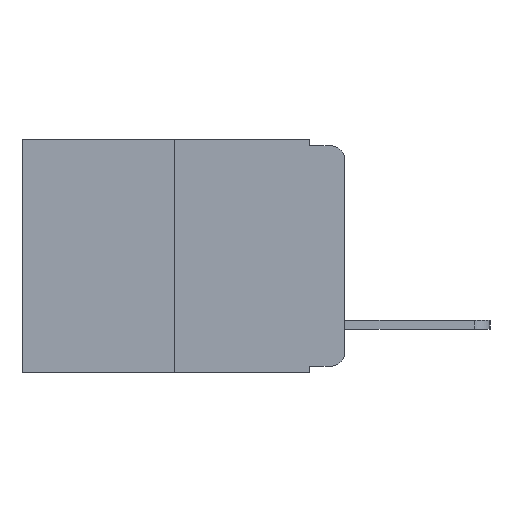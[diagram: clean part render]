
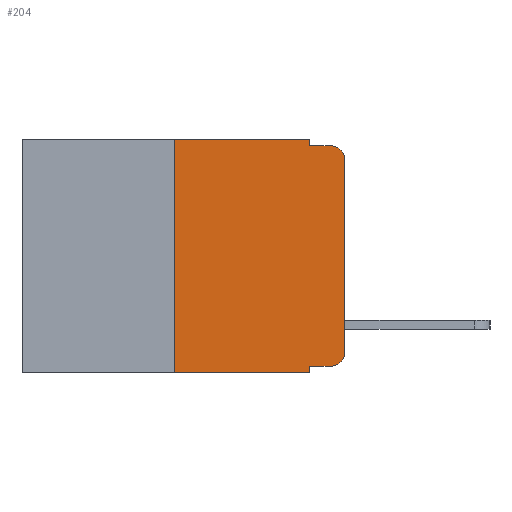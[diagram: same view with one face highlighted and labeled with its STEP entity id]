
A CAD part, left-side view. The second image highlights one B-rep face of the part: STEP entity #204.
In plain terms, the highlighted planar face has unit normal (-1, 0, 0).
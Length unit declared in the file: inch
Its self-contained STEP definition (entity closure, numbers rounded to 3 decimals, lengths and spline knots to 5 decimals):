
#204 = ADVANCED_FACE ( 'NONE', ( #9454 ), #4370, .F. ) ;
#456 = LINE ( 'NONE', #2460, #6495 ) ;
#551 = CARTESIAN_POINT ( 'NONE',  ( 0., 0.051, -0.333 ) ) ;
#660 = VERTEX_POINT ( 'NONE', #8153 ) ;
#873 = DIRECTION ( 'NONE',  ( 0., 0., -1. ) ) ;
#1065 = VERTEX_POINT ( 'NONE', #3341 ) ;
#1550 = VERTEX_POINT ( 'NONE', #4967 ) ;
#1679 = ORIENTED_EDGE ( 'NONE', *, *, #2929, .F. ) ;
#1696 = DIRECTION ( 'NONE',  ( -1., 0., 0. ) ) ;
#1979 = EDGE_CURVE ( 'NONE', #2777, #8733, #5225, .T. ) ;
#2117 = VECTOR ( 'NONE', #873, 39.37008 ) ;
#2119 = AXIS2_PLACEMENT_3D ( 'NONE', #10527, #1696, #3161 ) ;
#2141 = VECTOR ( 'NONE', #7348, 39.37008 ) ;
#2323 = VECTOR ( 'NONE', #13300, 39.37008 ) ;
#2385 = ORIENTED_EDGE ( 'NONE', *, *, #2818, .T. ) ;
#2408 = VERTEX_POINT ( 'NONE', #9678 ) ;
#2435 = VERTEX_POINT ( 'NONE', #3087 ) ;
#2460 = CARTESIAN_POINT ( 'NONE',  ( 0., 0.25, 0. ) ) ;
#2524 = AXIS2_PLACEMENT_3D ( 'NONE', #8845, #6250, #6197 ) ;
#2617 = LINE ( 'NONE', #12095, #13291 ) ;
#2777 = VERTEX_POINT ( 'NONE', #4160 ) ;
#2818 = EDGE_CURVE ( 'NONE', #9133, #2435, #13343, .T. ) ;
#2821 = EDGE_CURVE ( 'NONE', #5228, #9133, #7777, .T. ) ;
#2844 = EDGE_CURVE ( 'NONE', #5228, #1065, #8124, .T. ) ;
#2929 = EDGE_CURVE ( 'NONE', #6166, #2777, #456, .T. ) ;
#2976 = EDGE_CURVE ( 'NONE', #8733, #660, #5194, .T. ) ;
#3087 = CARTESIAN_POINT ( 'NONE',  ( 0., 0., -0.313 ) ) ;
#3161 = DIRECTION ( 'NONE',  ( 0., 0., -1. ) ) ;
#3341 = CARTESIAN_POINT ( 'NONE',  ( 0., 0.051, -0.343 ) ) ;
#3514 = EDGE_LOOP ( 'NONE', ( #6257, #3715, #9325, #4050, #9951, #1679, #7538, #12842, #7850, #2385 ) ) ;
#3715 = ORIENTED_EDGE ( 'NONE', *, *, #4859, .T. ) ;
#4050 = ORIENTED_EDGE ( 'NONE', *, *, #2976, .F. ) ;
#4076 = DIRECTION ( 'NONE',  ( 0., -1., 0. ) ) ;
#4118 = DIRECTION ( 'NONE',  ( 0., 0., -1. ) ) ;
#4160 = CARTESIAN_POINT ( 'NONE',  ( 0., 0.25, 0. ) ) ;
#4166 = CARTESIAN_POINT ( 'NONE',  ( 0., 0.051, 0. ) ) ;
#4370 = PLANE ( 'NONE',  #9123 ) ;
#4435 = VECTOR ( 'NONE', #9724, 39.37008 ) ;
#4780 = DIRECTION ( 'NONE',  ( 0., 0., 1. ) ) ;
#4843 = EDGE_CURVE ( 'NONE', #660, #1550, #9995, .T. ) ;
#4859 = EDGE_CURVE ( 'NONE', #2408, #1550, #12608, .T. ) ;
#4967 = CARTESIAN_POINT ( 'NONE',  ( 0., 0.02, -0.01 ) ) ;
#5015 = VECTOR ( 'NONE', #4076, 39.37008 ) ;
#5018 = EDGE_CURVE ( 'NONE', #2435, #2408, #2617, .T. ) ;
#5194 = LINE ( 'NONE', #6098, #2117 ) ;
#5225 = LINE ( 'NONE', #10826, #2141 ) ;
#5228 = VERTEX_POINT ( 'NONE', #551 ) ;
#5672 = DIRECTION ( 'NONE',  ( 0., 0., 1. ) ) ;
#5868 = DIRECTION ( 'NONE',  ( 0., 0., -1. ) ) ;
#5957 = CARTESIAN_POINT ( 'NONE',  ( 0., 0.051, 0. ) ) ;
#6098 = CARTESIAN_POINT ( 'NONE',  ( 0., 0.051, 0. ) ) ;
#6166 = VERTEX_POINT ( 'NONE', #12625 ) ;
#6197 = DIRECTION ( 'NONE',  ( 0., 0., -1. ) ) ;
#6250 = DIRECTION ( 'NONE',  ( -1., 0., 0. ) ) ;
#6257 = ORIENTED_EDGE ( 'NONE', *, *, #5018, .T. ) ;
#6495 = VECTOR ( 'NONE', #4780, 39.37008 ) ;
#7348 = DIRECTION ( 'NONE',  ( 0., -1., 0. ) ) ;
#7538 = ORIENTED_EDGE ( 'NONE', *, *, #8996, .T. ) ;
#7777 = LINE ( 'NONE', #10585, #5015 ) ;
#7850 = ORIENTED_EDGE ( 'NONE', *, *, #2821, .T. ) ;
#8124 = LINE ( 'NONE', #4166, #12781 ) ;
#8153 = CARTESIAN_POINT ( 'NONE',  ( 0., 0.051, -0.01 ) ) ;
#8733 = VERTEX_POINT ( 'NONE', #5957 ) ;
#8845 = CARTESIAN_POINT ( 'NONE',  ( 0., 0.02, -0.03 ) ) ;
#8996 = EDGE_CURVE ( 'NONE', #6166, #1065, #10521, .T. ) ;
#9123 = AXIS2_PLACEMENT_3D ( 'NONE', #9563, #9785, #5868 ) ;
#9133 = VERTEX_POINT ( 'NONE', #9452 ) ;
#9325 = ORIENTED_EDGE ( 'NONE', *, *, #4843, .F. ) ;
#9452 = CARTESIAN_POINT ( 'NONE',  ( 0., 0.02, -0.333 ) ) ;
#9454 = FACE_OUTER_BOUND ( 'NONE', #3514, .T. ) ;
#9563 = CARTESIAN_POINT ( 'NONE',  ( 0., 0.473, 0. ) ) ;
#9676 = CARTESIAN_POINT ( 'NONE',  ( 0., 0.051, -0.01 ) ) ;
#9678 = CARTESIAN_POINT ( 'NONE',  ( 0., 0., -0.03 ) ) ;
#9724 = DIRECTION ( 'NONE',  ( 0., -1., 0. ) ) ;
#9785 = DIRECTION ( 'NONE',  ( 1., 0., 0. ) ) ;
#9951 = ORIENTED_EDGE ( 'NONE', *, *, #1979, .F. ) ;
#9995 = LINE ( 'NONE', #9676, #4435 ) ;
#10276 = CARTESIAN_POINT ( 'NONE',  ( 0., 0.473, -0.343 ) ) ;
#10521 = LINE ( 'NONE', #10276, #2323 ) ;
#10527 = CARTESIAN_POINT ( 'NONE',  ( 0., 0.02, -0.313 ) ) ;
#10585 = CARTESIAN_POINT ( 'NONE',  ( 0., 0.051, -0.333 ) ) ;
#10826 = CARTESIAN_POINT ( 'NONE',  ( 0., 0.473, 0. ) ) ;
#12095 = CARTESIAN_POINT ( 'NONE',  ( 0., 0., 0. ) ) ;
#12608 = CIRCLE ( 'NONE', #2524, 0.02 ) ;
#12625 = CARTESIAN_POINT ( 'NONE',  ( 0., 0.25, -0.343 ) ) ;
#12781 = VECTOR ( 'NONE', #4118, 39.37008 ) ;
#12842 = ORIENTED_EDGE ( 'NONE', *, *, #2844, .F. ) ;
#13291 = VECTOR ( 'NONE', #5672, 39.37008 ) ;
#13300 = DIRECTION ( 'NONE',  ( 0., -1., 0. ) ) ;
#13343 = CIRCLE ( 'NONE', #2119, 0.02 ) ;
